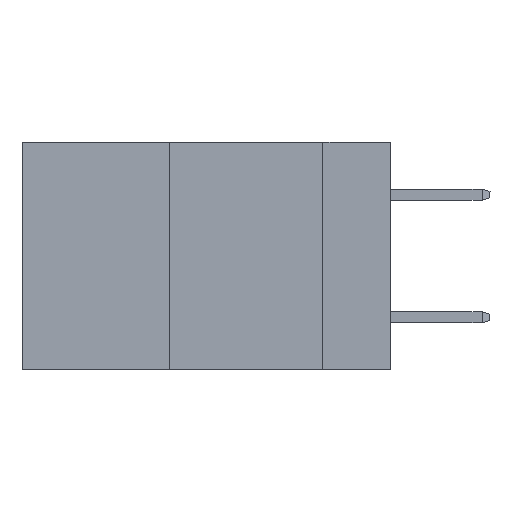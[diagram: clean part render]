
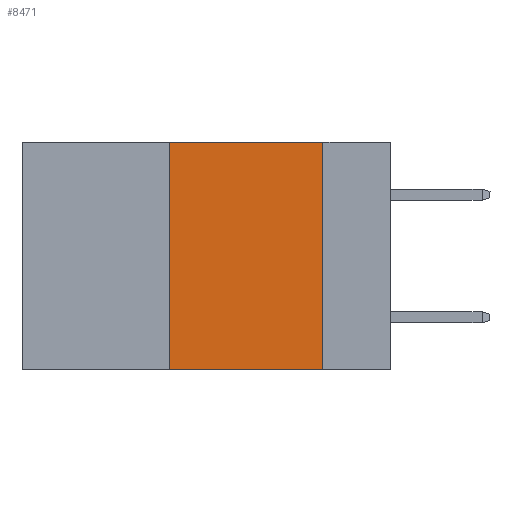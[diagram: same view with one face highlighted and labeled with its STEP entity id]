
A CAD part, left-side view. The second image highlights one B-rep face of the part: STEP entity #8471.
In plain terms, the highlighted planar face has unit normal (-1, 0, 0).
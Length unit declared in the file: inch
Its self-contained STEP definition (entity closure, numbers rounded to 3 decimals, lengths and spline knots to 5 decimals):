
#716 = CARTESIAN_POINT ( 'NONE',  ( 0., 0.36, 0. ) ) ;
#1124 = ORIENTED_EDGE ( 'NONE', *, *, #16094, .T. ) ;
#2390 = VERTEX_POINT ( 'NONE', #2631 ) ;
#2631 = CARTESIAN_POINT ( 'NONE',  ( 0., 0.11, 0. ) ) ;
#2970 = CARTESIAN_POINT ( 'NONE',  ( 0., 0.6, 0. ) ) ;
#3030 = EDGE_CURVE ( 'NONE', #2390, #8885, #3972, .T. ) ;
#3624 = AXIS2_PLACEMENT_3D ( 'NONE', #7111, #15692, #8310 ) ;
#3972 = LINE ( 'NONE', #10727, #11121 ) ;
#4300 = DIRECTION ( 'NONE',  ( 0., -1., 0. ) ) ;
#4730 = EDGE_CURVE ( 'NONE', #11142, #6390, #5096, .T. ) ;
#5096 = LINE ( 'NONE', #716, #11827 ) ;
#6353 = DIRECTION ( 'NONE',  ( 0., -1., 0. ) ) ;
#6390 = VERTEX_POINT ( 'NONE', #6408 ) ;
#6408 = CARTESIAN_POINT ( 'NONE',  ( 0., 0.36, 0. ) ) ;
#6469 = CARTESIAN_POINT ( 'NONE',  ( 0., 0.11, -0.37 ) ) ;
#7081 = FACE_OUTER_BOUND ( 'NONE', #13985, .T. ) ;
#7111 = CARTESIAN_POINT ( 'NONE',  ( 0., 0.6, 0. ) ) ;
#8310 = DIRECTION ( 'NONE',  ( 0., 0., -1. ) ) ;
#8471 = ADVANCED_FACE ( 'NONE', ( #7081 ), #14530, .F. ) ;
#8885 = VERTEX_POINT ( 'NONE', #6469 ) ;
#9354 = VECTOR ( 'NONE', #4300, 39.37008 ) ;
#9605 = VECTOR ( 'NONE', #6353, 39.37008 ) ;
#9687 = EDGE_CURVE ( 'NONE', #6390, #2390, #15845, .T. ) ;
#9700 = DIRECTION ( 'NONE',  ( 0., 0., 1. ) ) ;
#10594 = ORIENTED_EDGE ( 'NONE', *, *, #3030, .F. ) ;
#10727 = CARTESIAN_POINT ( 'NONE',  ( 0., 0.11, 0. ) ) ;
#11114 = DIRECTION ( 'NONE',  ( 0., 0., -1. ) ) ;
#11121 = VECTOR ( 'NONE', #11114, 39.37008 ) ;
#11142 = VERTEX_POINT ( 'NONE', #14772 ) ;
#11827 = VECTOR ( 'NONE', #9700, 39.37008 ) ;
#12545 = LINE ( 'NONE', #13858, #9605 ) ;
#13834 = ORIENTED_EDGE ( 'NONE', *, *, #9687, .F. ) ;
#13858 = CARTESIAN_POINT ( 'NONE',  ( 0., 0.6, -0.37 ) ) ;
#13985 = EDGE_LOOP ( 'NONE', ( #10594, #13834, #14210, #1124 ) ) ;
#14210 = ORIENTED_EDGE ( 'NONE', *, *, #4730, .F. ) ;
#14530 = PLANE ( 'NONE',  #3624 ) ;
#14772 = CARTESIAN_POINT ( 'NONE',  ( 0., 0.36, -0.37 ) ) ;
#15692 = DIRECTION ( 'NONE',  ( 1., 0., 0. ) ) ;
#15845 = LINE ( 'NONE', #2970, #9354 ) ;
#16094 = EDGE_CURVE ( 'NONE', #11142, #8885, #12545, .T. ) ;
